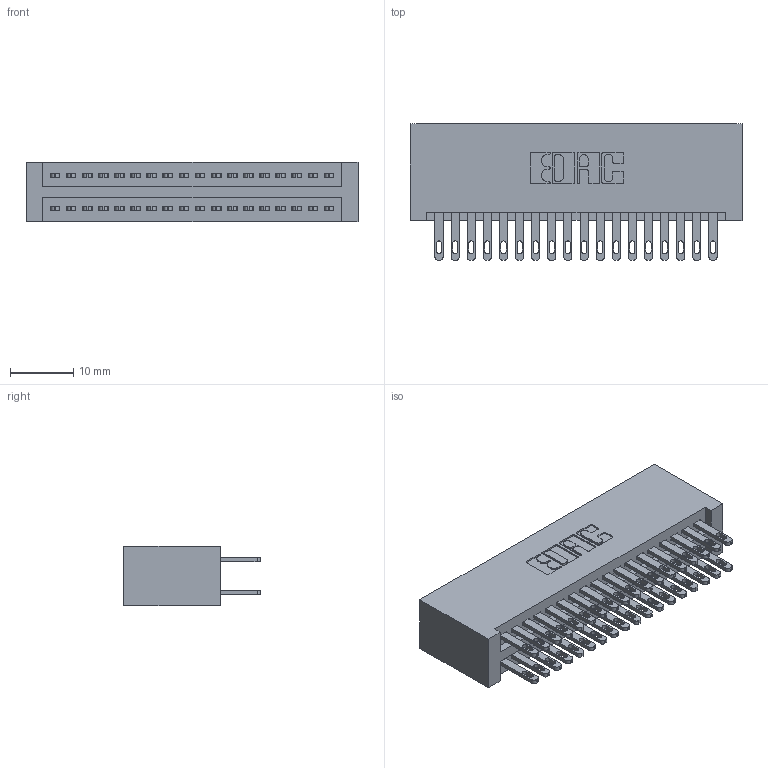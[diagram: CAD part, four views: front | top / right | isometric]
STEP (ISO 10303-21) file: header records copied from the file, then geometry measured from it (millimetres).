
FILE_DESCRIPTION (( 'STEP AP203' ), '1' );
FILE_NAME ('345-036-500-201.STEP', '2019-10-28T11:04:32', ( '' ), ( '' ), 'SwSTEP 2.0', 'SolidWorks 2016', '' );
FILE_SCHEMA (( 'CONFIG_CONTROL_DESIGN' ));
Length unit declared in the file: inch
Products named in the file (3): 345-036-500-201; 345-292-001_345-293-100; 345 Part_No Mounting Lugs
Assembly tree (37 placements, depth 2):
  345-036-500-201
    345 Part_No Mounting Lugs
    345-292-001_345-293-100  x36
Bounding box: 52.32 x 21.51 x 9.4 mm (x, y, z)
Volume: 5585.9 mm3; surface area: 8462.6 mm2
Topology: 37 solids, 37 shells, 1774 faces, 5393 edges, 3594 vertices
Faces by surface type: plane 1048, cylinder 726
Entity records: 17007 total; most frequent: CARTESIAN_POINT 2872, ORIENTED_EDGE 2806, DIRECTION 2559, EDGE_CURVE 1403, VECTOR 1203, LINE 1203, VERTEX_POINT 934, AXIS2_PLACEMENT_3D 678
